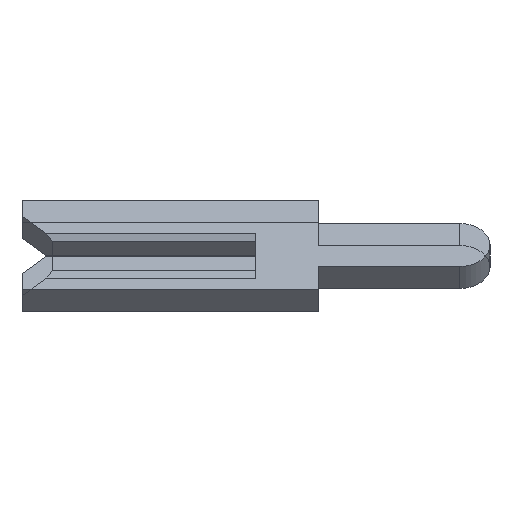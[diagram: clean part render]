
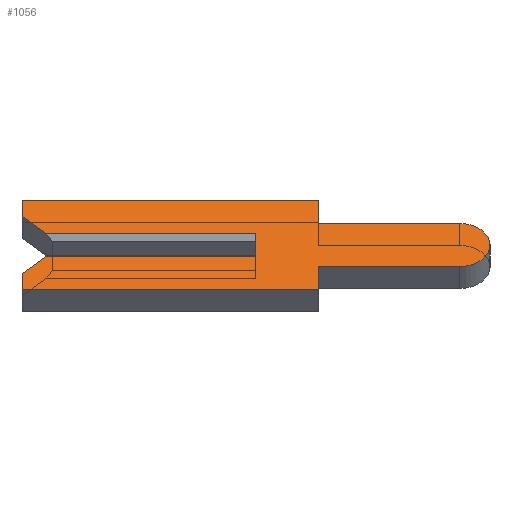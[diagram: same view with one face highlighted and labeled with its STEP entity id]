
A CAD part, left-side view. The second image highlights one B-rep face of the part: STEP entity #1056.
In plain terms, the highlighted face is planar.
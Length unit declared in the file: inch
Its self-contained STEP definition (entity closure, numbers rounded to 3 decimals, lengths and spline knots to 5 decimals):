
#4 = ORIENTED_EDGE ( 'NONE', *, *, #2142, .F. ) ;
#214 = VERTEX_POINT ( 'NONE', #1496 ) ;
#240 = CARTESIAN_POINT ( 'NONE',  ( -0.01, 0., 0.01 ) ) ;
#269 = LINE ( 'NONE', #2058, #376 ) ;
#294 = CARTESIAN_POINT ( 'NONE',  ( -0.01, -0.04, -0.0195 ) ) ;
#317 = LINE ( 'NONE', #859, #2093 ) ;
#320 = VECTOR ( 'NONE', #3330, 39.37008 ) ;
#374 = EDGE_CURVE ( 'NONE', #3359, #1317, #269, .T. ) ;
#376 = VECTOR ( 'NONE', #1145, 39.37008 ) ;
#396 = EDGE_CURVE ( 'NONE', #2442, #3359, #2743, .T. ) ;
#405 = EDGE_CURVE ( 'NONE', #2581, #3828, #1060, .T. ) ;
#421 = ORIENTED_EDGE ( 'NONE', *, *, #2939, .F. ) ;
#422 = VECTOR ( 'NONE', #456, 39.37008 ) ;
#456 = DIRECTION ( 'NONE',  ( 0., -1., 0. ) ) ;
#470 = LINE ( 'NONE', #3372, #515 ) ;
#481 = ORIENTED_EDGE ( 'NONE', *, *, #396, .F. ) ;
#515 = VECTOR ( 'NONE', #2406, 39.37008 ) ;
#525 = DIRECTION ( 'NONE',  ( 1., 0., 0. ) ) ;
#567 = VECTOR ( 'NONE', #3418, 39.37008 ) ;
#604 = CARTESIAN_POINT ( 'NONE',  ( -0.01, -0.04, -0.04 ) ) ;
#631 = ORIENTED_EDGE ( 'NONE', *, *, #1408, .F. ) ;
#719 = EDGE_CURVE ( 'NONE', #2841, #1721, #3280, .T. ) ;
#720 = LINE ( 'NONE', #912, #1998 ) ;
#763 = CARTESIAN_POINT ( 'NONE',  ( -0.01, 0.15, 0.04 ) ) ;
#768 = VERTEX_POINT ( 'NONE', #240 ) ;
#859 = CARTESIAN_POINT ( 'NONE',  ( -0.01, 0., 0.0065 ) ) ;
#912 = CARTESIAN_POINT ( 'NONE',  ( -0.01, 0.15, 0.026 ) ) ;
#954 = ORIENTED_EDGE ( 'NONE', *, *, #2907, .F. ) ;
#956 = CARTESIAN_POINT ( 'NONE',  ( -0.01, -0.04, 0.0195 ) ) ;
#1024 = CARTESIAN_POINT ( 'NONE',  ( -0.01, -0.1305, 0. ) ) ;
#1056 = ADVANCED_FACE ( 'NONE', ( #3620 ), #3621, .F. ) ;
#1060 = LINE ( 'NONE', #3629, #2199 ) ;
#1078 = VERTEX_POINT ( 'NONE', #2684 ) ;
#1145 = DIRECTION ( 'NONE',  ( 0., 0., -1. ) ) ;
#1161 = CARTESIAN_POINT ( 'NONE',  ( -0.01, -0.1305, 0.0195 ) ) ;
#1255 = EDGE_CURVE ( 'NONE', #1721, #214, #1914, .T. ) ;
#1317 = VERTEX_POINT ( 'NONE', #956 ) ;
#1351 = ORIENTED_EDGE ( 'NONE', *, *, #3384, .F. ) ;
#1370 = DIRECTION ( 'NONE',  ( 0., 0., -1. ) ) ;
#1408 = EDGE_CURVE ( 'NONE', #3828, #3245, #1814, .T. ) ;
#1485 = LINE ( 'NONE', #2787, #1586 ) ;
#1490 = CARTESIAN_POINT ( 'NONE',  ( -0.01, -0.1305, -0.0195 ) ) ;
#1496 = CARTESIAN_POINT ( 'NONE',  ( -0.01, -0.04, -0.04 ) ) ;
#1500 = CARTESIAN_POINT ( 'NONE',  ( -0.01, 0.15, -0.04 ) ) ;
#1515 = DIRECTION ( 'NONE',  ( 0., -1., 0. ) ) ;
#1586 = VECTOR ( 'NONE', #3085, 39.37008 ) ;
#1647 = CARTESIAN_POINT ( 'NONE',  ( -0.01, 0.134, -0.01 ) ) ;
#1721 = VERTEX_POINT ( 'NONE', #294 ) ;
#1814 = LINE ( 'NONE', #3732, #567 ) ;
#1882 = ORIENTED_EDGE ( 'NONE', *, *, #1255, .F. ) ;
#1914 = LINE ( 'NONE', #604, #2475 ) ;
#1928 = ORIENTED_EDGE ( 'NONE', *, *, #3837, .F. ) ;
#1957 = ORIENTED_EDGE ( 'NONE', *, *, #719, .F. ) ;
#1998 = VECTOR ( 'NONE', #2800, 39.37008 ) ;
#2058 = CARTESIAN_POINT ( 'NONE',  ( -0.01, -0.04, 0.04 ) ) ;
#2059 = VERTEX_POINT ( 'NONE', #3849 ) ;
#2083 = DIRECTION ( 'NONE',  ( 0., -1., 0. ) ) ;
#2093 = VECTOR ( 'NONE', #2116, 39.37008 ) ;
#2116 = DIRECTION ( 'NONE',  ( 0., 0., 1. ) ) ;
#2140 = VECTOR ( 'NONE', #3784, 39.37008 ) ;
#2142 = EDGE_CURVE ( 'NONE', #3073, #2841, #3426, .T. ) ;
#2198 = EDGE_LOOP ( 'NONE', ( #3932, #954, #631, #3767, #421, #1928, #1882, #1957, #4, #2258, #2597, #481, #1351, #3608 ) ) ;
#2199 = VECTOR ( 'NONE', #2997, 39.37008 ) ;
#2253 = DIRECTION ( 'NONE',  ( 1., 0., 0. ) ) ;
#2258 = ORIENTED_EDGE ( 'NONE', *, *, #2730, .F. ) ;
#2395 = CARTESIAN_POINT ( 'NONE',  ( -0.01, -0.04, 0.0195 ) ) ;
#2406 = DIRECTION ( 'NONE',  ( 0., 0., 1. ) ) ;
#2442 = VERTEX_POINT ( 'NONE', #2951 ) ;
#2461 = DIRECTION ( 'NONE',  ( 0., 0., -1. ) ) ;
#2475 = VECTOR ( 'NONE', #2758, 39.37008 ) ;
#2500 = LINE ( 'NONE', #3431, #422 ) ;
#2505 = CARTESIAN_POINT ( 'NONE',  ( -0.01, -0.04, 0.04 ) ) ;
#2552 = AXIS2_PLACEMENT_3D ( 'NONE', #3658, #525, #2461 ) ;
#2569 = AXIS2_PLACEMENT_3D ( 'NONE', #1024, #2253, #1370 ) ;
#2581 = VERTEX_POINT ( 'NONE', #3018 ) ;
#2597 = ORIENTED_EDGE ( 'NONE', *, *, #374, .F. ) ;
#2684 = CARTESIAN_POINT ( 'NONE',  ( -0.01, 0.15, 0.026 ) ) ;
#2692 = LINE ( 'NONE', #2395, #2937 ) ;
#2730 = EDGE_CURVE ( 'NONE', #1317, #3073, #2692, .T. ) ;
#2743 = LINE ( 'NONE', #763, #3432 ) ;
#2758 = DIRECTION ( 'NONE',  ( 0., 0., -1. ) ) ;
#2787 = CARTESIAN_POINT ( 'NONE',  ( -0.01, 0.1305, 0.0065 ) ) ;
#2800 = DIRECTION ( 'NONE',  ( 0., 0., 1. ) ) ;
#2830 = CARTESIAN_POINT ( 'NONE',  ( -0.01, 0.15, -0.04 ) ) ;
#2841 = VERTEX_POINT ( 'NONE', #1490 ) ;
#2907 = EDGE_CURVE ( 'NONE', #3245, #768, #317, .T. ) ;
#2937 = VECTOR ( 'NONE', #1515, 39.37008 ) ;
#2939 = EDGE_CURVE ( 'NONE', #2974, #2581, #470, .T. ) ;
#2951 = CARTESIAN_POINT ( 'NONE',  ( -0.01, 0.15, 0.04 ) ) ;
#2974 = VERTEX_POINT ( 'NONE', #1500 ) ;
#2997 = DIRECTION ( 'NONE',  ( 0., -0.707, 0.707 ) ) ;
#3000 = CARTESIAN_POINT ( 'NONE',  ( -0.01, 0., -0.01 ) ) ;
#3018 = CARTESIAN_POINT ( 'NONE',  ( -0.01, 0.15, -0.026 ) ) ;
#3025 = CARTESIAN_POINT ( 'NONE',  ( -0.01, -0.04, -0.0195 ) ) ;
#3044 = EDGE_CURVE ( 'NONE', #2059, #768, #2500, .T. ) ;
#3073 = VERTEX_POINT ( 'NONE', #1161 ) ;
#3085 = DIRECTION ( 'NONE',  ( 0., 0.707, 0.707 ) ) ;
#3245 = VERTEX_POINT ( 'NONE', #3000 ) ;
#3280 = LINE ( 'NONE', #3025, #320 ) ;
#3330 = DIRECTION ( 'NONE',  ( 0., 1., 0. ) ) ;
#3349 = EDGE_CURVE ( 'NONE', #2059, #1078, #1485, .T. ) ;
#3359 = VERTEX_POINT ( 'NONE', #2505 ) ;
#3372 = CARTESIAN_POINT ( 'NONE',  ( -0.01, 0.15, -0.026 ) ) ;
#3384 = EDGE_CURVE ( 'NONE', #1078, #2442, #720, .T. ) ;
#3418 = DIRECTION ( 'NONE',  ( 0., -1., 0. ) ) ;
#3426 = CIRCLE ( 'NONE', #2569, 0.0195 ) ;
#3431 = CARTESIAN_POINT ( 'NONE',  ( -0.01, 0.15, 0.01 ) ) ;
#3432 = VECTOR ( 'NONE', #2083, 39.37008 ) ;
#3608 = ORIENTED_EDGE ( 'NONE', *, *, #3349, .F. ) ;
#3620 = FACE_OUTER_BOUND ( 'NONE', #2198, .T. ) ;
#3621 = PLANE ( 'NONE',  #2552 ) ;
#3629 = CARTESIAN_POINT ( 'NONE',  ( -0.01, 0.1305, -0.0065 ) ) ;
#3658 = CARTESIAN_POINT ( 'NONE',  ( -0.01, -0.1305, 0. ) ) ;
#3732 = CARTESIAN_POINT ( 'NONE',  ( -0.01, -0.1305, -0.01 ) ) ;
#3767 = ORIENTED_EDGE ( 'NONE', *, *, #405, .F. ) ;
#3784 = DIRECTION ( 'NONE',  ( 0., 1., 0. ) ) ;
#3828 = VERTEX_POINT ( 'NONE', #1647 ) ;
#3837 = EDGE_CURVE ( 'NONE', #214, #2974, #3921, .T. ) ;
#3849 = CARTESIAN_POINT ( 'NONE',  ( -0.01, 0.134, 0.01 ) ) ;
#3921 = LINE ( 'NONE', #2830, #2140 ) ;
#3932 = ORIENTED_EDGE ( 'NONE', *, *, #3044, .T. ) ;
